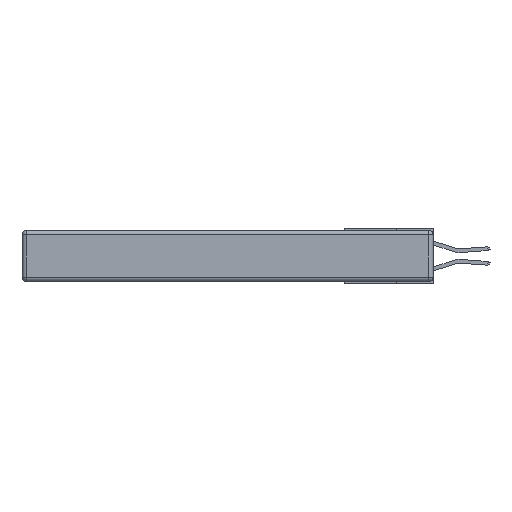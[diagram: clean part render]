
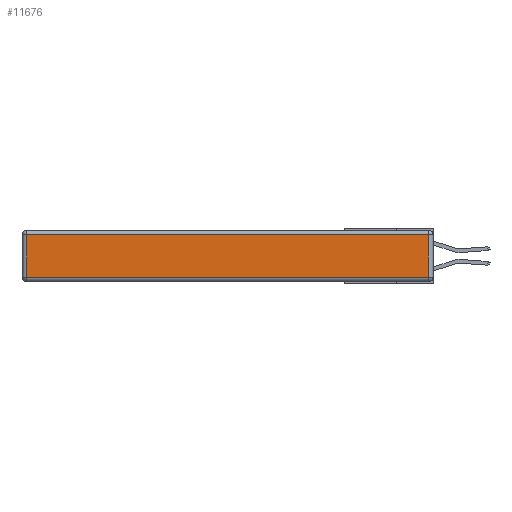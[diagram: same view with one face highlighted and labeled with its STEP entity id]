
A CAD part, left-side view. The second image highlights one B-rep face of the part: STEP entity #11676.
In plain terms, the highlighted planar face has unit normal (-1, 0, 0).
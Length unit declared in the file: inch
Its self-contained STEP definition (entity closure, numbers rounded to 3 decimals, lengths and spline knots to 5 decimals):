
#1655 = CARTESIAN_POINT ( 'NONE',  ( 0., 2.75, -0.03 ) ) ;
#3112 = LINE ( 'NONE', #11627, #14020 ) ;
#3416 = VECTOR ( 'NONE', #6265, 39.37008 ) ;
#3743 = CARTESIAN_POINT ( 'NONE',  ( 0., 2.72, -0.313 ) ) ;
#4029 = ORIENTED_EDGE ( 'NONE', *, *, #6741, .T. ) ;
#4717 = FACE_OUTER_BOUND ( 'NONE', #17076, .T. ) ;
#4993 = DIRECTION ( 'NONE',  ( 0., -1., 0. ) ) ;
#5681 = LINE ( 'NONE', #15786, #13255 ) ;
#6265 = DIRECTION ( 'NONE',  ( 0., 0., -1. ) ) ;
#6441 = DIRECTION ( 'NONE',  ( 0., 0., 1. ) ) ;
#6741 = EDGE_CURVE ( 'NONE', #15945, #16944, #8196, .T. ) ;
#7013 = VECTOR ( 'NONE', #15296, 39.37008 ) ;
#7269 = VERTEX_POINT ( 'NONE', #16322 ) ;
#7383 = EDGE_CURVE ( 'NONE', #12710, #7269, #5681, .T. ) ;
#8139 = CARTESIAN_POINT ( 'NONE',  ( 0., 0., -0.343 ) ) ;
#8196 = LINE ( 'NONE', #10153, #3416 ) ;
#8927 = ORIENTED_EDGE ( 'NONE', *, *, #11587, .T. ) ;
#8942 = ORIENTED_EDGE ( 'NONE', *, *, #7383, .T. ) ;
#9502 = EDGE_CURVE ( 'NONE', #16944, #12710, #3112, .T. ) ;
#10153 = CARTESIAN_POINT ( 'NONE',  ( 0., 2.72, -0.343 ) ) ;
#11278 = AXIS2_PLACEMENT_3D ( 'NONE', #8139, #15270, #11348 ) ;
#11348 = DIRECTION ( 'NONE',  ( 0., 0., 1. ) ) ;
#11587 = EDGE_CURVE ( 'NONE', #7269, #15945, #15423, .T. ) ;
#11627 = CARTESIAN_POINT ( 'NONE',  ( 0., 0., -0.313 ) ) ;
#11676 = ADVANCED_FACE ( 'NONE', ( #4717 ), #15102, .T. ) ;
#12710 = VERTEX_POINT ( 'NONE', #14612 ) ;
#13109 = ORIENTED_EDGE ( 'NONE', *, *, #9502, .T. ) ;
#13255 = VECTOR ( 'NONE', #6441, 39.37008 ) ;
#14020 = VECTOR ( 'NONE', #4993, 39.37008 ) ;
#14612 = CARTESIAN_POINT ( 'NONE',  ( 0., 0.03, -0.313 ) ) ;
#15102 = PLANE ( 'NONE',  #11278 ) ;
#15270 = DIRECTION ( 'NONE',  ( -1., 0., 0. ) ) ;
#15296 = DIRECTION ( 'NONE',  ( 0., 1., 0. ) ) ;
#15423 = LINE ( 'NONE', #1655, #7013 ) ;
#15786 = CARTESIAN_POINT ( 'NONE',  ( 0., 0.03, -0.343 ) ) ;
#15945 = VERTEX_POINT ( 'NONE', #17044 ) ;
#16322 = CARTESIAN_POINT ( 'NONE',  ( 0., 0.03, -0.03 ) ) ;
#16944 = VERTEX_POINT ( 'NONE', #3743 ) ;
#17044 = CARTESIAN_POINT ( 'NONE',  ( 0., 2.72, -0.03 ) ) ;
#17076 = EDGE_LOOP ( 'NONE', ( #13109, #8942, #8927, #4029 ) ) ;
